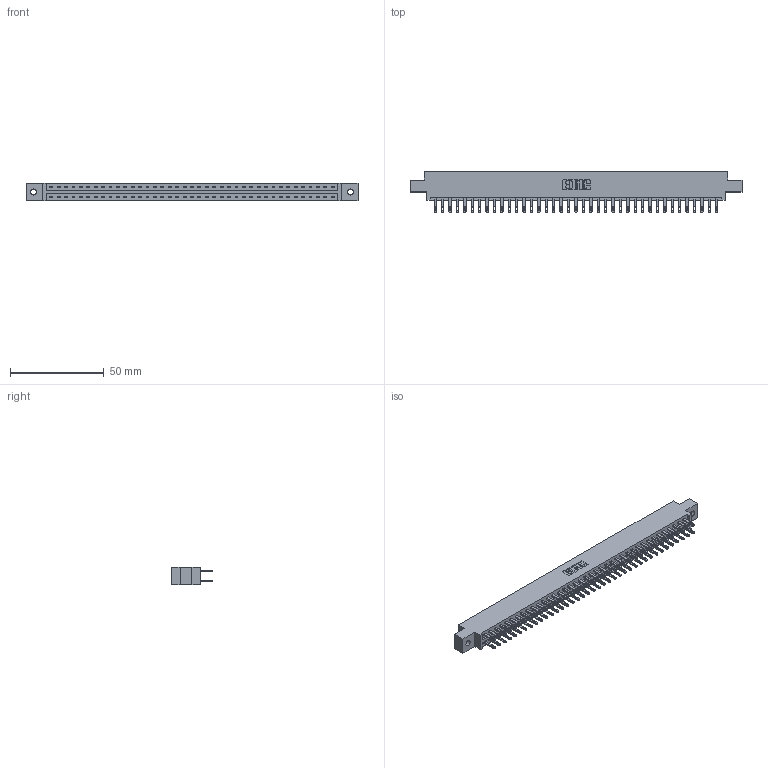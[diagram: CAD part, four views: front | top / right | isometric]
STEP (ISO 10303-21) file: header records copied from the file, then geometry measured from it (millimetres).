
FILE_DESCRIPTION (( 'STEP AP203' ), '1' );
FILE_NAME ('887-078-500-802.STEP', '2020-09-21T04:09:57', ( '' ), ( '' ), 'SwSTEP 2.0', 'SolidWorks 2020', '' );
FILE_SCHEMA (( 'CONFIG_CONTROL_DESIGN' ));
Length unit declared in the file: inch
Products named in the file (3): 837 Part_0.170 Offset - 0.128 Dia; 887-078-500-802; 345-292-001_345-293-100
Assembly tree (79 placements, depth 2):
  887-078-500-802
    837 Part_0.170 Offset - 0.128 Dia
    345-292-001_345-293-100  x78
Bounding box: 177.55 x 21.85 x 9.4 mm (x, y, z)
Volume: 18755.4 mm3; surface area: 21874.5 mm2
Topology: 79 solids, 79 shells, 4018 faces, 12257 edges, 8170 vertices
Faces by surface type: plane 2570, cylinder 1448
Entity records: 30691 total; most frequent: CARTESIAN_POINT 5174, ORIENTED_EDGE 5110, DIRECTION 4407, EDGE_CURVE 2555, LINE 2423, VECTOR 2423, VERTEX_POINT 1702, AXIS2_PLACEMENT_3D 992
